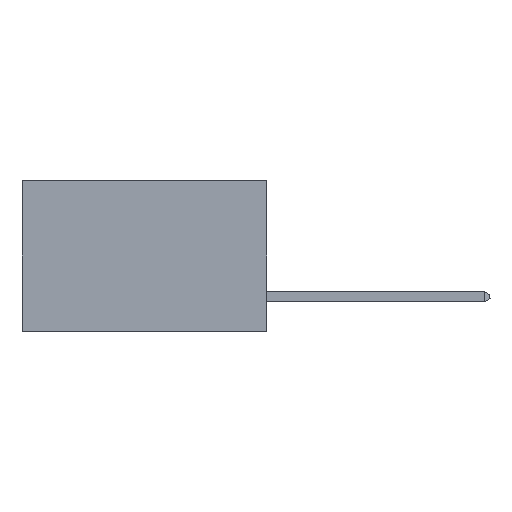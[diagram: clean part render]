
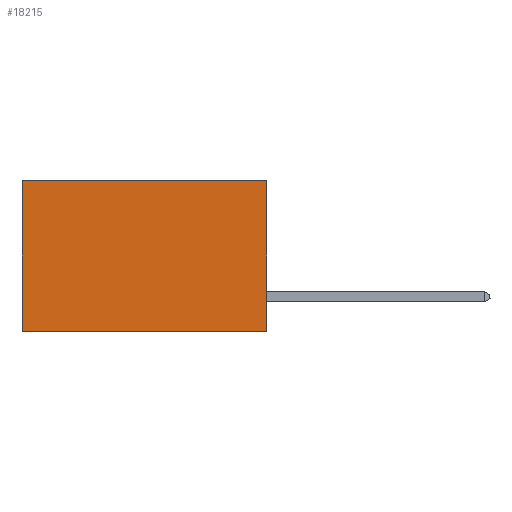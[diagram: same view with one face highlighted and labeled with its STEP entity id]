
A CAD part, left-side view. The second image highlights one B-rep face of the part: STEP entity #18215.
In plain terms, the highlighted planar face has unit normal (-1, 0, 0).
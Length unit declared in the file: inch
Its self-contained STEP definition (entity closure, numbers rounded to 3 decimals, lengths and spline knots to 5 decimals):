
#485 = DIRECTION ( 'NONE',  ( 0., 1., 0. ) ) ;
#921 = CARTESIAN_POINT ( 'NONE',  ( 0.2875, 0.6, 0. ) ) ;
#1836 = CARTESIAN_POINT ( 'NONE',  ( 0.2875, 0., 0. ) ) ;
#2182 = DIRECTION ( 'NONE',  ( 0., 1., 0. ) ) ;
#2432 = AXIS2_PLACEMENT_3D ( 'NONE', #28687, #2567, #13281 ) ;
#2567 = DIRECTION ( 'NONE',  ( 1., 0., 0. ) ) ;
#3278 = FACE_OUTER_BOUND ( 'NONE', #13206, .T. ) ;
#4584 = DIRECTION ( 'NONE',  ( 0., 0., -1. ) ) ;
#4667 = EDGE_CURVE ( 'NONE', #26618, #9311, #25678, .T. ) ;
#6615 = ORIENTED_EDGE ( 'NONE', *, *, #16883, .T. ) ;
#9311 = VERTEX_POINT ( 'NONE', #33140 ) ;
#9318 = VERTEX_POINT ( 'NONE', #25124 ) ;
#13206 = EDGE_LOOP ( 'NONE', ( #20064, #23073, #28370, #6615 ) ) ;
#13281 = DIRECTION ( 'NONE',  ( 0., 0., -1. ) ) ;
#14134 = EDGE_CURVE ( 'NONE', #18891, #9318, #24315, .T. ) ;
#15940 = VECTOR ( 'NONE', #2182, 39.37008 ) ;
#16883 = EDGE_CURVE ( 'NONE', #26618, #18891, #30696, .T. ) ;
#17532 = CARTESIAN_POINT ( 'NONE',  ( 0.2875, 0., 0. ) ) ;
#18184 = VECTOR ( 'NONE', #19703, 39.37008 ) ;
#18215 = ADVANCED_FACE ( 'NONE', ( #3278 ), #33706, .F. ) ;
#18891 = VERTEX_POINT ( 'NONE', #28537 ) ;
#19703 = DIRECTION ( 'NONE',  ( 0., 0., -1. ) ) ;
#20064 = ORIENTED_EDGE ( 'NONE', *, *, #14134, .T. ) ;
#23073 = ORIENTED_EDGE ( 'NONE', *, *, #28296, .F. ) ;
#23242 = CARTESIAN_POINT ( 'NONE',  ( 0.2875, 0., 0. ) ) ;
#24315 = LINE ( 'NONE', #921, #18184 ) ;
#24858 = VECTOR ( 'NONE', #4584, 39.37008 ) ;
#25124 = CARTESIAN_POINT ( 'NONE',  ( 0.2875, 0.6, -0.37 ) ) ;
#25678 = LINE ( 'NONE', #17532, #24858 ) ;
#26618 = VERTEX_POINT ( 'NONE', #23242 ) ;
#28296 = EDGE_CURVE ( 'NONE', #9311, #9318, #28573, .T. ) ;
#28370 = ORIENTED_EDGE ( 'NONE', *, *, #4667, .F. ) ;
#28537 = CARTESIAN_POINT ( 'NONE',  ( 0.2875, 0.6, 0. ) ) ;
#28573 = LINE ( 'NONE', #32230, #31862 ) ;
#28687 = CARTESIAN_POINT ( 'NONE',  ( 0.2875, 0., 0. ) ) ;
#30696 = LINE ( 'NONE', #1836, #15940 ) ;
#31862 = VECTOR ( 'NONE', #485, 39.37008 ) ;
#32230 = CARTESIAN_POINT ( 'NONE',  ( 0.2875, 0., -0.37 ) ) ;
#33140 = CARTESIAN_POINT ( 'NONE',  ( 0.2875, 0., -0.37 ) ) ;
#33706 = PLANE ( 'NONE',  #2432 ) ;
